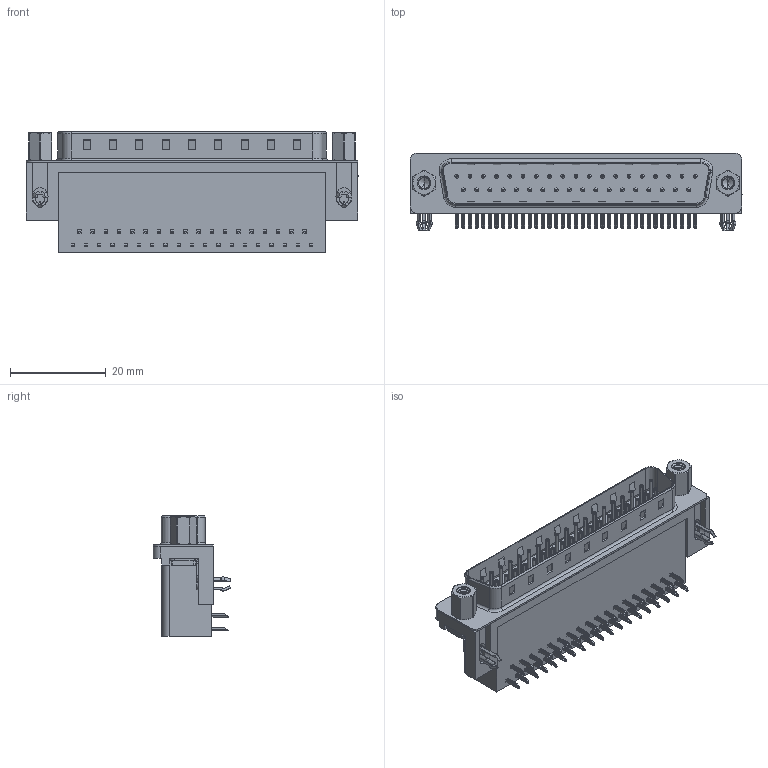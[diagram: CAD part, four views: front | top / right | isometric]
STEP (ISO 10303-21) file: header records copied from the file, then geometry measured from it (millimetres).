
FILE_DESCRIPTION (( 'STEP AP203' ), '1' );
FILE_NAME ('625-037-662-043.STEP', '2018-11-06T06:41:50', ( '' ), ( '' ), 'SwSTEP 2.0', 'SolidWorks 2016', '' );
FILE_SCHEMA (( 'CONFIG_CONTROL_DESIGN' ));
Length unit declared in the file: millimetre
Products named in the file (8): 625 Shell_37 Socket; 625 Contact Bottom; 625 Contact Top; 625 3 Prong Board Lock; 625 4-40 Threaded Rivet; 625 4-40 Hex Standoff 5; 625-037-662-043; 625 Housing_37 Socket
Assembly tree (45 placements, depth 2):
  625-037-662-043
    625 Housing_37 Socket
    625 Shell_37 Socket
    625 Contact Bottom  x18
    625 Contact Top  x19
    625 3 Prong Board Lock  x2
    625 4-40 Threaded Rivet  x2
    625 4-40 Hex Standoff 5  x2
Bounding box: 69.4 x 16.25 x 25.16 mm (x, y, z)
Volume: 12822.5 mm3; surface area: 12297.9 mm2
Topology: 45 solids, 45 shells, 3431 faces, 8565 edges, 5305 vertices
Faces by surface type: plane 2073, cylinder 995, torus 277, cone 68, bspline 18
Entity records: 33416 total; most frequent: CARTESIAN_POINT 9393, DIRECTION 4631, ORIENTED_EDGE 4562, EDGE_CURVE 2281, VECTOR 1545, LINE 1545, AXIS2_PLACEMENT_3D 1543, VERTEX_POINT 1474
